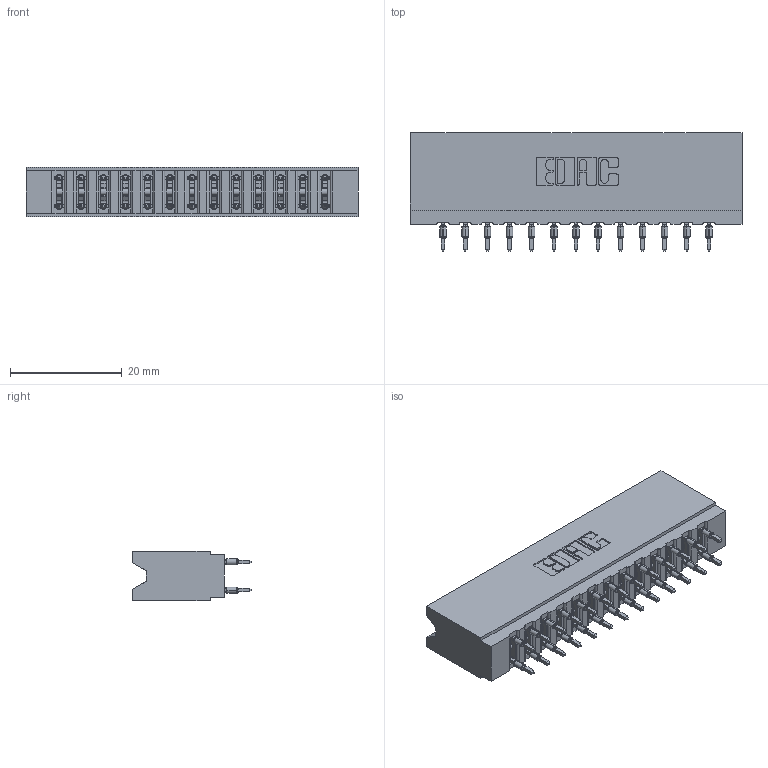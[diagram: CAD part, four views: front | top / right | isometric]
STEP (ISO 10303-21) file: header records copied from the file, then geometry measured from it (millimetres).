
FILE_DESCRIPTION (( 'STEP AP203' ), '1' );
FILE_NAME ('737-026-560-206.STEP', '2026-03-05T22:04:09', ( '' ), ( '' ), 'SwSTEP 2.0', 'SolidWorks 2023', '' );
FILE_SCHEMA (( 'CONFIG_CONTROL_DESIGN' ));
Length unit declared in the file: millimetre
Products named in the file (3): 737 Part_Insulator Option - 06; 737-026-560-206; 745-292-001_560
Assembly tree (27 placements, depth 2):
  737-026-560-206
    737 Part_Insulator Option - 06
    745-292-001_560  x26
Bounding box: 59.39 x 21.22 x 8.89 mm (x, y, z)
Volume: 6068.8 mm3; surface area: 9008.1 mm2
Topology: 27 solids, 27 shells, 2669 faces, 7303 edges, 4642 vertices
Faces by surface type: plane 1394, cylinder 599, bspline 520, torus 156
Entity records: 26584 total; most frequent: CARTESIAN_POINT 5128, ORIENTED_EDGE 4506, DIRECTION 3963, EDGE_CURVE 2253, VECTOR 1985, LINE 1985, VERTEX_POINT 1442, AXIS2_PLACEMENT_3D 989
